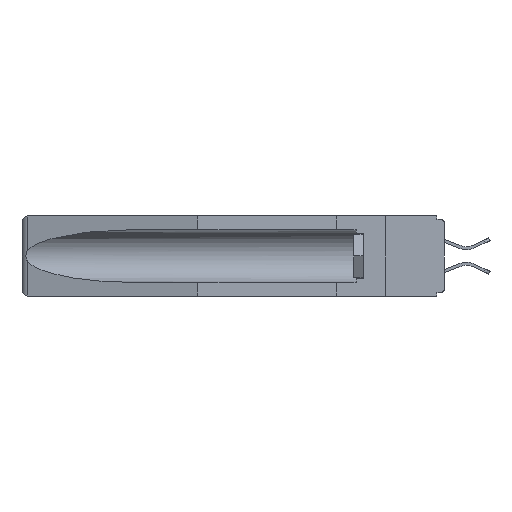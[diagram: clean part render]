
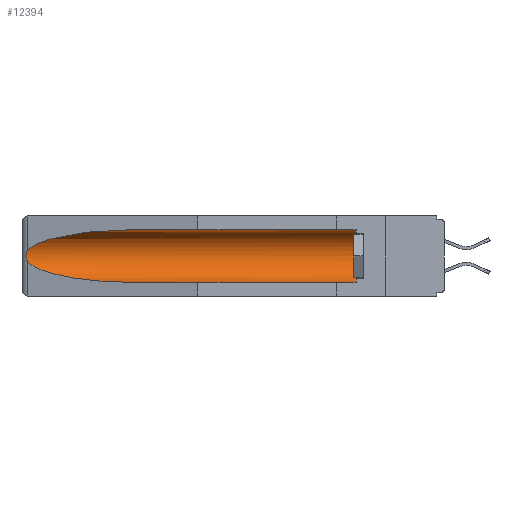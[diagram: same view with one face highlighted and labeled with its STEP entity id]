
A CAD part, left-side view. The second image highlights one B-rep face of the part: STEP entity #12394.
In plain terms, the highlighted cylindrical face has radius 2.857 mm (diameter 5.715 mm), a partial arc.
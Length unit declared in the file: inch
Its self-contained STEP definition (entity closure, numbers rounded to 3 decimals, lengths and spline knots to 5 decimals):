
#104 = CARTESIAN_POINT ( 'NONE',  ( 0.155, 1.07973, -0.059 ) ) ;
#122 = CARTESIAN_POINT ( 'NONE',  ( 0.155, -0.30754, -0.1715 ) ) ;
#269 = ORIENTED_EDGE ( 'NONE', *, *, #12220, .T. ) ;
#438 = VERTEX_POINT ( 'NONE', #18491 ) ;
#842 = CARTESIAN_POINT ( 'NONE',  ( 0.25451, 1.48313, -0.24835 ) ) ;
#1392 = CARTESIAN_POINT ( 'NONE',  ( 0.26597, 1.52961, -0.15275 ) ) ;
#1445 = AXIS2_PLACEMENT_3D ( 'NONE', #122, #2141, #2060 ) ;
#2001 = CARTESIAN_POINT ( 'NONE',  ( 0.155, 0.126, -0.059 ) ) ;
#2060 = DIRECTION ( 'NONE',  ( 0., 0., 1. ) ) ;
#2082 = CARTESIAN_POINT ( 'NONE',  ( 0.25451, 1.48313, -0.09465 ) ) ;
#2141 = DIRECTION ( 'NONE',  ( 0., 1., 0. ) ) ;
#2731 = VERTEX_POINT ( 'NONE', #23225 ) ;
#2935 =( BOUNDED_CURVE ( )  B_SPLINE_CURVE ( 3, ( #17537, #21399, #2082, #19559 ),
 .UNSPECIFIED., .F., .T. ) 
 B_SPLINE_CURVE_WITH_KNOTS ( ( 4, 4 ),
 ( 4.71239, 6.08839 ),
 .UNSPECIFIED. ) 
 CURVE ( )  GEOMETRIC_REPRESENTATION_ITEM ( )  RATIONAL_B_SPLINE_CURVE ( ( 1., 0.848, 0.848, 1. ) ) 
 REPRESENTATION_ITEM ( '' )  );
#3407 = LINE ( 'NONE', #10694, #18888 ) ;
#3592 = CARTESIAN_POINT ( 'NONE',  ( 0.26654, 1.53092, -0.15636 ) ) ;
#5314 = EDGE_CURVE ( 'NONE', #2731, #438, #12013, .T. ) ;
#5542 = CARTESIAN_POINT ( 'NONE',  ( 0.2673, 1.5327, -0.16383 ) ) ;
#7038 = CYLINDRICAL_SURFACE ( 'NONE', #1445, 0.1125 ) ;
#7489 = CARTESIAN_POINT ( 'NONE',  ( 0.155, 0.126, -0.284 ) ) ;
#9039 = ORIENTED_EDGE ( 'NONE', *, *, #9501, .T. ) ;
#9501 = EDGE_CURVE ( 'NONE', #438, #15839, #20943, .T. ) ;
#9868 = AXIS2_PLACEMENT_3D ( 'NONE', #24235, #10886, #14471 ) ;
#10117 = CARTESIAN_POINT ( 'NONE',  ( 0.155, -0.30754, -0.284 ) ) ;
#10140 = CIRCLE ( 'NONE', #9868, 0.1125 ) ;
#10284 = VERTEX_POINT ( 'NONE', #2001 ) ;
#10694 = CARTESIAN_POINT ( 'NONE',  ( 0.155, -0.30754, -0.059 ) ) ;
#10886 = DIRECTION ( 'NONE',  ( 0., -1., 0. ) ) ;
#11083 = CARTESIAN_POINT ( 'NONE',  ( 0.26597, 1.5296, -0.19026 ) ) ;
#11093 = CARTESIAN_POINT ( 'NONE',  ( 0.155, 1.07973, -0.284 ) ) ;
#11358 = ORIENTED_EDGE ( 'NONE', *, *, #21449, .T. ) ;
#11930 = EDGE_LOOP ( 'NONE', ( #20340, #14574, #9039, #13587, #11358, #269 ) ) ;
#12013 = B_SPLINE_CURVE_WITH_KNOTS ( 'NONE', 3,
 ( #14995, #1392, #3592, #5542, #24612, #19217, #19046, #24692, #11083, #20969 ),
 .UNSPECIFIED., .F., .F.,
 ( 4, 2, 2, 2, 4 ),
 ( 0., 0.00029, 0.00058, 0.00087, 0.00117 ),
 .UNSPECIFIED. ) ;
#12220 = EDGE_CURVE ( 'NONE', #10284, #17017, #3407, .T. ) ;
#12394 = ADVANCED_FACE ( 'NONE', ( #14652 ), #7038, .F. ) ;
#13548 = VECTOR ( 'NONE', #15897, 39.37008 ) ;
#13587 = ORIENTED_EDGE ( 'NONE', *, *, #20206, .F. ) ;
#14436 = CARTESIAN_POINT ( 'NONE',  ( 0.21114, 1.30732, -0.284 ) ) ;
#14471 = DIRECTION ( 'NONE',  ( 0., 0., 1. ) ) ;
#14574 = ORIENTED_EDGE ( 'NONE', *, *, #5314, .T. ) ;
#14652 = FACE_OUTER_BOUND ( 'NONE', #11930, .T. ) ;
#14923 = VERTEX_POINT ( 'NONE', #7489 ) ;
#14995 = CARTESIAN_POINT ( 'NONE',  ( 0.26537, 1.52718, -0.14972 ) ) ;
#15839 = VERTEX_POINT ( 'NONE', #11093 ) ;
#15897 = DIRECTION ( 'NONE',  ( 0., 1., 0. ) ) ;
#16041 = EDGE_CURVE ( 'NONE', #17017, #2731, #2935, .T. ) ;
#16381 = CARTESIAN_POINT ( 'NONE',  ( 0.155, 1.07973, -0.284 ) ) ;
#17017 = VERTEX_POINT ( 'NONE', #104 ) ;
#17537 = CARTESIAN_POINT ( 'NONE',  ( 0.155, 1.07973, -0.059 ) ) ;
#18491 = CARTESIAN_POINT ( 'NONE',  ( 0.26537, 1.52718, -0.19328 ) ) ;
#18888 = VECTOR ( 'NONE', #24278, 39.37008 ) ;
#19046 = CARTESIAN_POINT ( 'NONE',  ( 0.2673, 1.53269, -0.17917 ) ) ;
#19217 = CARTESIAN_POINT ( 'NONE',  ( 0.2675, 1.53308, -0.17534 ) ) ;
#19559 = CARTESIAN_POINT ( 'NONE',  ( 0.26537, 1.52718, -0.14972 ) ) ;
#20206 = EDGE_CURVE ( 'NONE', #14923, #15839, #21081, .T. ) ;
#20340 = ORIENTED_EDGE ( 'NONE', *, *, #16041, .T. ) ;
#20943 =( BOUNDED_CURVE ( )  B_SPLINE_CURVE ( 3, ( #24284, #842, #14436, #16381 ),
 .UNSPECIFIED., .F., .F. ) 
 B_SPLINE_CURVE_WITH_KNOTS ( ( 4, 4 ),
 ( 0.1948, 1.5708 ),
 .UNSPECIFIED. ) 
 CURVE ( )  GEOMETRIC_REPRESENTATION_ITEM ( )  RATIONAL_B_SPLINE_CURVE ( ( 1., 0.848, 0.848, 1. ) ) 
 REPRESENTATION_ITEM ( '' )  );
#20969 = CARTESIAN_POINT ( 'NONE',  ( 0.26537, 1.52718, -0.19328 ) ) ;
#21081 = LINE ( 'NONE', #10117, #13548 ) ;
#21399 = CARTESIAN_POINT ( 'NONE',  ( 0.21114, 1.30732, -0.059 ) ) ;
#21449 = EDGE_CURVE ( 'NONE', #14923, #10284, #10140, .T. ) ;
#23225 = CARTESIAN_POINT ( 'NONE',  ( 0.26537, 1.52718, -0.14972 ) ) ;
#24235 = CARTESIAN_POINT ( 'NONE',  ( 0.155, 0.126, -0.1715 ) ) ;
#24278 = DIRECTION ( 'NONE',  ( 0., 1., 0. ) ) ;
#24284 = CARTESIAN_POINT ( 'NONE',  ( 0.26537, 1.52718, -0.19328 ) ) ;
#24612 = CARTESIAN_POINT ( 'NONE',  ( 0.2675, 1.53308, -0.16763 ) ) ;
#24692 = CARTESIAN_POINT ( 'NONE',  ( 0.26655, 1.53094, -0.18657 ) ) ;
